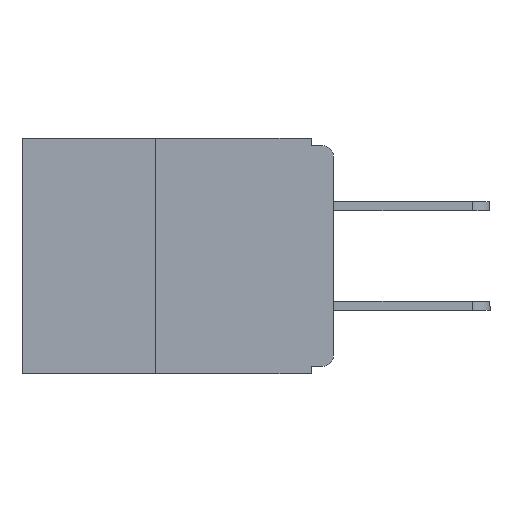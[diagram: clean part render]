
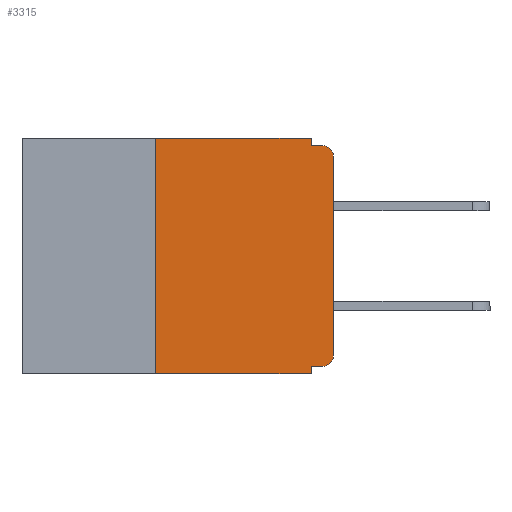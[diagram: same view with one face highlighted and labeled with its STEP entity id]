
A CAD part, left-side view. The second image highlights one B-rep face of the part: STEP entity #3315.
In plain terms, the highlighted planar face has unit normal (-1, 0, 0).
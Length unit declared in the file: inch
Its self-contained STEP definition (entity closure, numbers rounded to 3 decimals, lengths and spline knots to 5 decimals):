
#503 = ORIENTED_EDGE ( 'NONE', *, *, #12685, .T. ) ;
#530 = AXIS2_PLACEMENT_3D ( 'NONE', #4357, #3887, #3851 ) ;
#544 = ORIENTED_EDGE ( 'NONE', *, *, #11996, .T. ) ;
#867 = ORIENTED_EDGE ( 'NONE', *, *, #13050, .F. ) ;
#874 = LINE ( 'NONE', #6760, #1287 ) ;
#966 = EDGE_CURVE ( 'NONE', #7792, #12535, #4590, .T. ) ;
#967 = VERTEX_POINT ( 'NONE', #12950 ) ;
#1080 = VECTOR ( 'NONE', #7772, 39.37008 ) ;
#1287 = VECTOR ( 'NONE', #7111, 39.37008 ) ;
#1636 = ORIENTED_EDGE ( 'NONE', *, *, #4581, .F. ) ;
#1783 = ORIENTED_EDGE ( 'NONE', *, *, #966, .F. ) ;
#1844 = ORIENTED_EDGE ( 'NONE', *, *, #4563, .F. ) ;
#1873 = ORIENTED_EDGE ( 'NONE', *, *, #4496, .T. ) ;
#2056 = LINE ( 'NONE', #7430, #1080 ) ;
#2103 = AXIS2_PLACEMENT_3D ( 'NONE', #10400, #10301, #10278 ) ;
#2141 = ORIENTED_EDGE ( 'NONE', *, *, #4468, .F. ) ;
#2157 = ORIENTED_EDGE ( 'NONE', *, *, #12146, .F. ) ;
#2176 = ORIENTED_EDGE ( 'NONE', *, *, #11788, .T. ) ;
#2387 = VECTOR ( 'NONE', #9040, 39.37008 ) ;
#2401 = LINE ( 'NONE', #9053, #2387 ) ;
#2976 = VERTEX_POINT ( 'NONE', #10378 ) ;
#3023 = VECTOR ( 'NONE', #9383, 39.37008 ) ;
#3307 = VECTOR ( 'NONE', #4428, 39.37008 ) ;
#3315 = ADVANCED_FACE ( 'NONE', ( #4452 ), #4275, .F. ) ;
#3449 = LINE ( 'NONE', #4589, #3307 ) ;
#3567 = LINE ( 'NONE', #9555, #3023 ) ;
#3851 = DIRECTION ( 'NONE',  ( 0., 0., -1. ) ) ;
#3887 = DIRECTION ( 'NONE',  ( 1., 0., 0. ) ) ;
#3951 = VECTOR ( 'NONE', #9844, 39.37008 ) ;
#4275 = PLANE ( 'NONE',  #530 ) ;
#4328 = LINE ( 'NONE', #10020, #3951 ) ;
#4357 = CARTESIAN_POINT ( 'NONE',  ( 0., 0.437, 0. ) ) ;
#4391 = CARTESIAN_POINT ( 'NONE',  ( 0., 0.015, -0.32 ) ) ;
#4428 = DIRECTION ( 'NONE',  ( 0., 0., 1. ) ) ;
#4452 = FACE_OUTER_BOUND ( 'NONE', #11883, .T. ) ;
#4468 = EDGE_CURVE ( 'NONE', #10487, #7129, #4328, .T. ) ;
#4496 = EDGE_CURVE ( 'NONE', #2976, #7129, #3567, .T. ) ;
#4512 = VERTEX_POINT ( 'NONE', #8790 ) ;
#4563 = EDGE_CURVE ( 'NONE', #2976, #7792, #2056, .T. ) ;
#4581 = EDGE_CURVE ( 'NONE', #12535, #4512, #874, .T. ) ;
#4584 = VECTOR ( 'NONE', #12859, 39.37008 ) ;
#4589 = CARTESIAN_POINT ( 'NONE',  ( 0., 0., 0. ) ) ;
#4590 = LINE ( 'NONE', #10877, #4584 ) ;
#5069 = CARTESIAN_POINT ( 'NONE',  ( 0., 0.031, -0.33 ) ) ;
#5139 = DIRECTION ( 'NONE',  ( 0., 1., 0. ) ) ;
#5182 = CARTESIAN_POINT ( 'NONE',  ( 0., 0., -0.32 ) ) ;
#5214 = VECTOR ( 'NONE', #5139, 39.37008 ) ;
#5274 = LINE ( 'NONE', #5182, #5214 ) ;
#5727 = CIRCLE ( 'NONE', #8215, 0.015 ) ;
#6140 = CARTESIAN_POINT ( 'NONE',  ( 0., 0., -0.025 ) ) ;
#6305 = CIRCLE ( 'NONE', #2103, 0.015 ) ;
#6760 = CARTESIAN_POINT ( 'NONE',  ( 0., 0.031, 0. ) ) ;
#7111 = DIRECTION ( 'NONE',  ( 0., 0., -1. ) ) ;
#7129 = VERTEX_POINT ( 'NONE', #5069 ) ;
#7407 = DIRECTION ( 'NONE',  ( 0., 0., -1. ) ) ;
#7430 = CARTESIAN_POINT ( 'NONE',  ( 0., 0.25, -0.33 ) ) ;
#7443 = DIRECTION ( 'NONE',  ( -1., 0., 0. ) ) ;
#7536 = CARTESIAN_POINT ( 'NONE',  ( 0., 0.015, -0.025 ) ) ;
#7772 = DIRECTION ( 'NONE',  ( 0., 0., 1. ) ) ;
#7792 = VERTEX_POINT ( 'NONE', #9791 ) ;
#7878 = CARTESIAN_POINT ( 'NONE',  ( 0., 0., -0.305 ) ) ;
#8215 = AXIS2_PLACEMENT_3D ( 'NONE', #7536, #7443, #7407 ) ;
#8790 = CARTESIAN_POINT ( 'NONE',  ( 0., 0.031, -0.01 ) ) ;
#8853 = VERTEX_POINT ( 'NONE', #7878 ) ;
#9040 = DIRECTION ( 'NONE',  ( 0., -1., 0. ) ) ;
#9053 = CARTESIAN_POINT ( 'NONE',  ( 0., 0., -0.01 ) ) ;
#9149 = VERTEX_POINT ( 'NONE', #4391 ) ;
#9383 = DIRECTION ( 'NONE',  ( 0., -1., 0. ) ) ;
#9555 = CARTESIAN_POINT ( 'NONE',  ( 0., 0.437, -0.33 ) ) ;
#9569 = CARTESIAN_POINT ( 'NONE',  ( 0., 0.031, 0. ) ) ;
#9791 = CARTESIAN_POINT ( 'NONE',  ( 0., 0.25, 0. ) ) ;
#9844 = DIRECTION ( 'NONE',  ( 0., 0., -1. ) ) ;
#10020 = CARTESIAN_POINT ( 'NONE',  ( 0., 0.031, -0.33 ) ) ;
#10278 = DIRECTION ( 'NONE',  ( 0., 0., -1. ) ) ;
#10301 = DIRECTION ( 'NONE',  ( -1., 0., 0. ) ) ;
#10378 = CARTESIAN_POINT ( 'NONE',  ( 0., 0.25, -0.33 ) ) ;
#10400 = CARTESIAN_POINT ( 'NONE',  ( 0., 0.015, -0.305 ) ) ;
#10487 = VERTEX_POINT ( 'NONE', #11824 ) ;
#10877 = CARTESIAN_POINT ( 'NONE',  ( 0., 0.437, 0. ) ) ;
#11788 = EDGE_CURVE ( 'NONE', #9149, #8853, #6305, .T. ) ;
#11824 = CARTESIAN_POINT ( 'NONE',  ( 0., 0.031, -0.32 ) ) ;
#11883 = EDGE_LOOP ( 'NONE', ( #503, #544, #867, #1636, #1783, #1844, #1873, #2141, #2157, #2176 ) ) ;
#11996 = EDGE_CURVE ( 'NONE', #12107, #967, #5727, .T. ) ;
#12107 = VERTEX_POINT ( 'NONE', #6140 ) ;
#12146 = EDGE_CURVE ( 'NONE', #9149, #10487, #5274, .T. ) ;
#12535 = VERTEX_POINT ( 'NONE', #9569 ) ;
#12685 = EDGE_CURVE ( 'NONE', #8853, #12107, #3449, .T. ) ;
#12859 = DIRECTION ( 'NONE',  ( 0., -1., 0. ) ) ;
#12950 = CARTESIAN_POINT ( 'NONE',  ( 0., 0.015, -0.01 ) ) ;
#13050 = EDGE_CURVE ( 'NONE', #4512, #967, #2401, .T. ) ;
